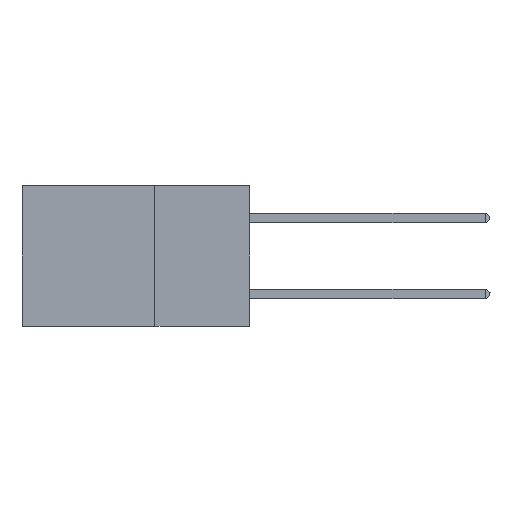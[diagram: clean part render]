
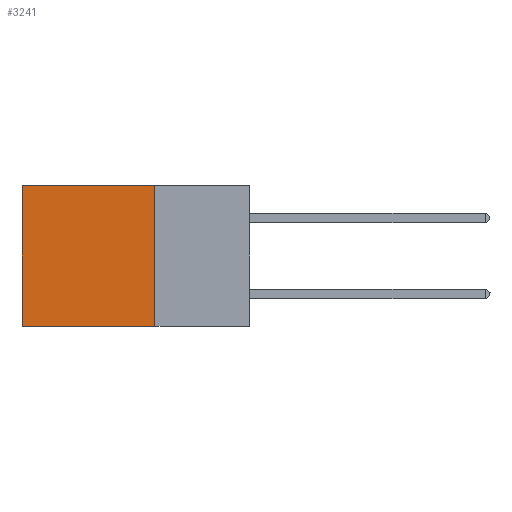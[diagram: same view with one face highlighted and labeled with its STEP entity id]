
A CAD part, left-side view. The second image highlights one B-rep face of the part: STEP entity #3241.
In plain terms, the highlighted planar face has unit normal (-1, 0, 0).
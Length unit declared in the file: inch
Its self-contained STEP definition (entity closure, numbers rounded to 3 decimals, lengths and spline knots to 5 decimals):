
#173 = ORIENTED_EDGE ( 'NONE', *, *, #22612, .F. ) ;
#618 = LINE ( 'NONE', #1255, #1518 ) ;
#854 = LINE ( 'NONE', #15399, #4786 ) ;
#1167 = CARTESIAN_POINT ( 'NONE',  ( 0.2875, 0.6, 0. ) ) ;
#1255 = CARTESIAN_POINT ( 'NONE',  ( 0.2875, 0.25, 0. ) ) ;
#1446 = EDGE_CURVE ( 'NONE', #20902, #19604, #854, .T. ) ;
#1518 = VECTOR ( 'NONE', #16808, 39.37008 ) ;
#2969 = LINE ( 'NONE', #13669, #18164 ) ;
#3241 = ADVANCED_FACE ( 'NONE', ( #6449 ), #23413, .F. ) ;
#4783 = EDGE_CURVE ( 'NONE', #20902, #6815, #618, .T. ) ;
#4786 = VECTOR ( 'NONE', #19912, 39.37008 ) ;
#6366 = EDGE_CURVE ( 'NONE', #6815, #21746, #2969, .T. ) ;
#6449 = FACE_OUTER_BOUND ( 'NONE', #10984, .T. ) ;
#6815 = VERTEX_POINT ( 'NONE', #1167 ) ;
#7732 = DIRECTION ( 'NONE',  ( 0., 0., -1. ) ) ;
#8470 = ORIENTED_EDGE ( 'NONE', *, *, #1446, .F. ) ;
#10071 = ORIENTED_EDGE ( 'NONE', *, *, #6366, .T. ) ;
#10221 = CARTESIAN_POINT ( 'NONE',  ( 0.2875, 0.6, -0.37 ) ) ;
#10984 = EDGE_LOOP ( 'NONE', ( #10071, #173, #8470, #23839 ) ) ;
#11287 = AXIS2_PLACEMENT_3D ( 'NONE', #23584, #18400, #16500 ) ;
#11884 = VECTOR ( 'NONE', #16927, 39.37008 ) ;
#13117 = LINE ( 'NONE', #24770, #11884 ) ;
#13639 = CARTESIAN_POINT ( 'NONE',  ( 0.2875, 0.25, -0.37 ) ) ;
#13669 = CARTESIAN_POINT ( 'NONE',  ( 0.2875, 0.6, 0. ) ) ;
#15399 = CARTESIAN_POINT ( 'NONE',  ( 0.2875, 0.25, 0. ) ) ;
#16500 = DIRECTION ( 'NONE',  ( 0., 0., -1. ) ) ;
#16808 = DIRECTION ( 'NONE',  ( 0., 1., 0. ) ) ;
#16927 = DIRECTION ( 'NONE',  ( 0., 1., 0. ) ) ;
#18164 = VECTOR ( 'NONE', #7732, 39.37008 ) ;
#18400 = DIRECTION ( 'NONE',  ( 1., 0., 0. ) ) ;
#19518 = CARTESIAN_POINT ( 'NONE',  ( 0.2875, 0.25, 0. ) ) ;
#19604 = VERTEX_POINT ( 'NONE', #13639 ) ;
#19912 = DIRECTION ( 'NONE',  ( 0., 0., -1. ) ) ;
#20902 = VERTEX_POINT ( 'NONE', #19518 ) ;
#21746 = VERTEX_POINT ( 'NONE', #10221 ) ;
#22612 = EDGE_CURVE ( 'NONE', #19604, #21746, #13117, .T. ) ;
#23413 = PLANE ( 'NONE',  #11287 ) ;
#23584 = CARTESIAN_POINT ( 'NONE',  ( 0.2875, 0.25, 0. ) ) ;
#23839 = ORIENTED_EDGE ( 'NONE', *, *, #4783, .T. ) ;
#24770 = CARTESIAN_POINT ( 'NONE',  ( 0.2875, 0.25, -0.37 ) ) ;
